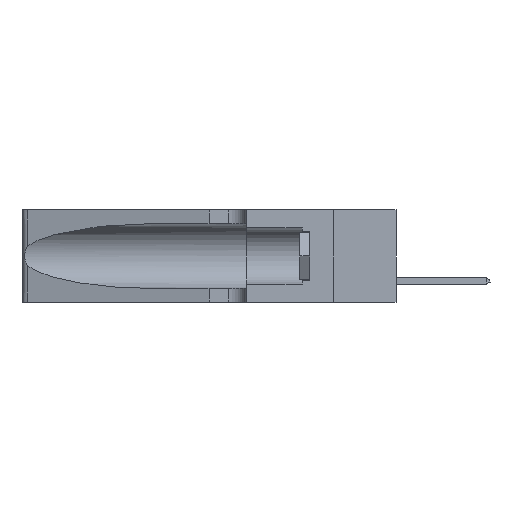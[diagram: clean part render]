
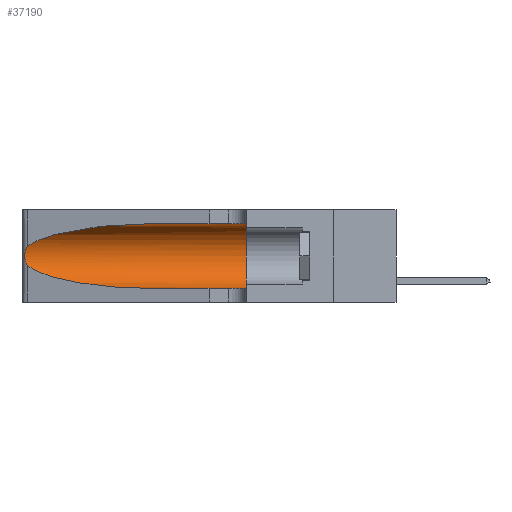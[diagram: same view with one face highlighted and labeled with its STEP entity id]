
A CAD part, left-side view. The second image highlights one B-rep face of the part: STEP entity #37190.
In plain terms, the highlighted cylindrical face has radius 3.308 mm (diameter 6.617 mm), a partial arc.
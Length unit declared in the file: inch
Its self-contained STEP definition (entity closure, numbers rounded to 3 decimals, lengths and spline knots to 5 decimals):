
#451 = CARTESIAN_POINT ( 'NONE',  ( 0.1305, 0.72297, 0.05475 ) ) ;
#617 = CARTESIAN_POINT ( 'NONE',  ( 0.26018, 1.23835, 0.19895 ) ) ;
#878 = VERTEX_POINT ( 'NONE', #4616 ) ;
#1417 = CARTESIAN_POINT ( 'NONE',  ( 0.25639, 1.23186, 0.15144 ) ) ;
#2430 = VERTEX_POINT ( 'NONE', #11079 ) ;
#3741 = CARTESIAN_POINT ( 'NONE',  ( 0.25639, 1.23184, 0.21858 ) ) ;
#3812 =( BOUNDED_CURVE ( )  B_SPLINE_CURVE ( 3, ( #35145, #16982, #20317, #14401 ),
 .UNSPECIFIED., .F., .F. ) 
 B_SPLINE_CURVE_WITH_KNOTS ( ( 4, 4 ),
 ( 3.44316, 4.71239 ),
 .UNSPECIFIED. ) 
 CURVE ( )  GEOMETRIC_REPRESENTATION_ITEM ( )  RATIONAL_B_SPLINE_CURVE ( ( 1., 0.87, 0.87, 1. ) ) 
 REPRESENTATION_ITEM ( '' )  );
#4048 = CARTESIAN_POINT ( 'NONE',  ( 0.1305, 0.72297, 0.31525 ) ) ;
#4404 = CARTESIAN_POINT ( 'NONE',  ( 0.25487, 1.22718, 0.14631 ) ) ;
#4616 = CARTESIAN_POINT ( 'NONE',  ( 0.1305, 0.35, 0.05475 ) ) ;
#4811 = CARTESIAN_POINT ( 'NONE',  ( 0.25789, 1.23486, 0.15765 ) ) ;
#5491 = EDGE_CURVE ( 'NONE', #2430, #9729, #37933, .T. ) ;
#6852 = FACE_OUTER_BOUND ( 'NONE', #16888, .T. ) ;
#7353 = DIRECTION ( 'NONE',  ( 0., 0., -1. ) ) ;
#7369 = CARTESIAN_POINT ( 'NONE',  ( 0.25787, 1.23484, 0.2124 ) ) ;
#9101 = CIRCLE ( 'NONE', #20072, 0.13025 ) ;
#9484 = CARTESIAN_POINT ( 'NONE',  ( 0.1305, 1.61858, 0.31525 ) ) ;
#9729 = VERTEX_POINT ( 'NONE', #17830 ) ;
#10604 = ORIENTED_EDGE ( 'NONE', *, *, #14417, .T. ) ;
#10691 = DIRECTION ( 'NONE',  ( 0., -1., 0. ) ) ;
#11079 = CARTESIAN_POINT ( 'NONE',  ( 0.1305, 0.72297, 0.31525 ) ) ;
#11424 = CARTESIAN_POINT ( 'NONE',  ( 0.1305, 1.61858, 0.05475 ) ) ;
#11961 = ORIENTED_EDGE ( 'NONE', *, *, #31995, .T. ) ;
#14401 = CARTESIAN_POINT ( 'NONE',  ( 0.1305, 0.72297, 0.05475 ) ) ;
#14417 = EDGE_CURVE ( 'NONE', #2430, #28086, #16423, .T. ) ;
#16423 =( BOUNDED_CURVE ( )  B_SPLINE_CURVE ( 3, ( #4048, #16458, #31931, #25172 ),
 .UNSPECIFIED., .F., .F. ) 
 B_SPLINE_CURVE_WITH_KNOTS ( ( 4, 4 ),
 ( 1.5708, 2.84003 ),
 .UNSPECIFIED. ) 
 CURVE ( )  GEOMETRIC_REPRESENTATION_ITEM ( )  RATIONAL_B_SPLINE_CURVE ( ( 1., 0.87, 0.87, 1. ) ) 
 REPRESENTATION_ITEM ( '' )  );
#16458 = CARTESIAN_POINT ( 'NONE',  ( 0.18966, 0.96281, 0.31525 ) ) ;
#16888 = EDGE_LOOP ( 'NONE', ( #10604, #11961, #30677, #17256, #26706, #29489 ) ) ;
#16982 = CARTESIAN_POINT ( 'NONE',  ( 0.2373, 1.15595, 0.08982 ) ) ;
#17066 = EDGE_CURVE ( 'NONE', #9729, #878, #9101, .T. ) ;
#17219 = CARTESIAN_POINT ( 'NONE',  ( 0.25555, 1.22993, 0.14849 ) ) ;
#17256 = ORIENTED_EDGE ( 'NONE', *, *, #33440, .T. ) ;
#17830 = CARTESIAN_POINT ( 'NONE',  ( 0.1305, 0.35, 0.31525 ) ) ;
#18504 = LINE ( 'NONE', #11424, #37282 ) ;
#19630 = CARTESIAN_POINT ( 'NONE',  ( 0.25555, 1.22994, 0.2215 ) ) ;
#19884 = CARTESIAN_POINT ( 'NONE',  ( 0.26017, 1.23833, 0.17102 ) ) ;
#20072 = AXIS2_PLACEMENT_3D ( 'NONE', #37763, #39904, #27528 ) ;
#20317 = CARTESIAN_POINT ( 'NONE',  ( 0.18966, 0.96281, 0.05475 ) ) ;
#20432 = VERTEX_POINT ( 'NONE', #451 ) ;
#21503 = AXIS2_PLACEMENT_3D ( 'NONE', #26044, #10691, #7353 ) ;
#22171 = CARTESIAN_POINT ( 'NONE',  ( 0.26075, 1.23896, 0.19203 ) ) ;
#22989 = VECTOR ( 'NONE', #34934, 39.37008 ) ;
#25172 = CARTESIAN_POINT ( 'NONE',  ( 0.25487, 1.22718, 0.22369 ) ) ;
#26044 = CARTESIAN_POINT ( 'NONE',  ( 0.1305, 1.61858, 0.185 ) ) ;
#26706 = ORIENTED_EDGE ( 'NONE', *, *, #17066, .F. ) ;
#27119 = CYLINDRICAL_SURFACE ( 'NONE', #21503, 0.13025 ) ;
#27528 = DIRECTION ( 'NONE',  ( 0., 0., 1. ) ) ;
#28086 = VERTEX_POINT ( 'NONE', #28468 ) ;
#28468 = CARTESIAN_POINT ( 'NONE',  ( 0.25487, 1.22718, 0.22369 ) ) ;
#28792 = CARTESIAN_POINT ( 'NONE',  ( 0.25487, 1.22718, 0.22369 ) ) ;
#28998 = B_SPLINE_CURVE_WITH_KNOTS ( 'NONE', 3,
 ( #28792, #19630, #3741, #7369, #34432, #617, #22171, #31499, #19884, #32408, #4811, #1417, #17219, #4404 ),
 .UNSPECIFIED., .F., .F.,
 ( 4, 2, 2, 2, 2, 2, 4 ),
 ( 0., 0.00027, 0.00053, 0.00107, 0.0016, 0.00187, 0.00214 ),
 .UNSPECIFIED. ) ;
#29489 = ORIENTED_EDGE ( 'NONE', *, *, #5491, .F. ) ;
#29638 = DIRECTION ( 'NONE',  ( 0., -1., 0. ) ) ;
#30677 = ORIENTED_EDGE ( 'NONE', *, *, #33327, .T. ) ;
#31499 = CARTESIAN_POINT ( 'NONE',  ( 0.26075, 1.23896, 0.178 ) ) ;
#31931 = CARTESIAN_POINT ( 'NONE',  ( 0.2373, 1.15595, 0.28018 ) ) ;
#31995 = EDGE_CURVE ( 'NONE', #28086, #37328, #28998, .T. ) ;
#32408 = CARTESIAN_POINT ( 'NONE',  ( 0.25856, 1.23593, 0.16098 ) ) ;
#33327 = EDGE_CURVE ( 'NONE', #37328, #20432, #3812, .T. ) ;
#33440 = EDGE_CURVE ( 'NONE', #20432, #878, #18504, .T. ) ;
#34432 = CARTESIAN_POINT ( 'NONE',  ( 0.25854, 1.2359, 0.20912 ) ) ;
#34934 = DIRECTION ( 'NONE',  ( 0., -1., 0. ) ) ;
#35145 = CARTESIAN_POINT ( 'NONE',  ( 0.25487, 1.22718, 0.14631 ) ) ;
#37190 = ADVANCED_FACE ( 'NONE', ( #6852 ), #27119, .F. ) ;
#37282 = VECTOR ( 'NONE', #29638, 39.37008 ) ;
#37328 = VERTEX_POINT ( 'NONE', #39012 ) ;
#37763 = CARTESIAN_POINT ( 'NONE',  ( 0.1305, 0.35, 0.185 ) ) ;
#37933 = LINE ( 'NONE', #9484, #22989 ) ;
#39012 = CARTESIAN_POINT ( 'NONE',  ( 0.25487, 1.22718, 0.14631 ) ) ;
#39904 = DIRECTION ( 'NONE',  ( 0., 1., 0. ) ) ;
